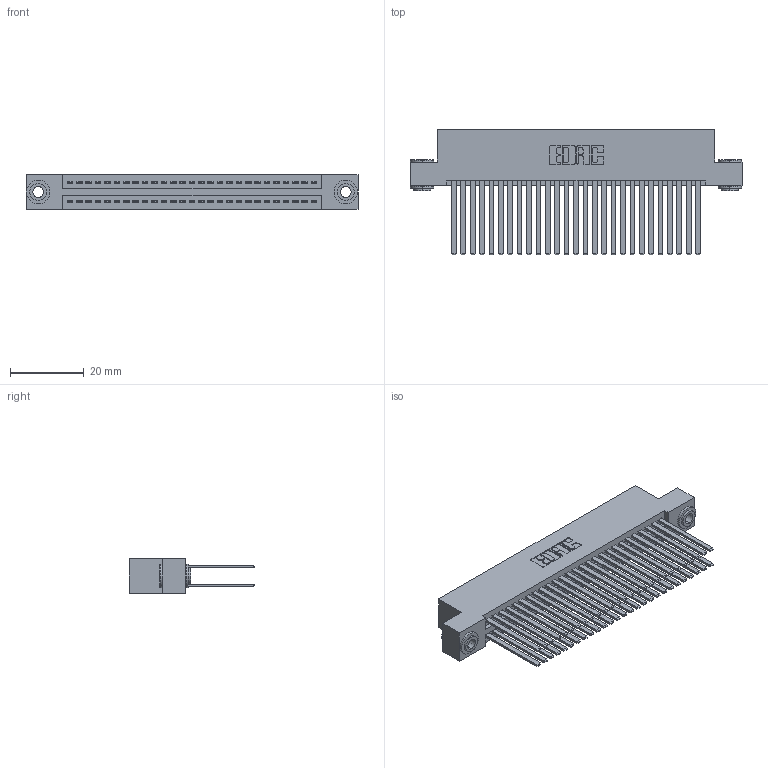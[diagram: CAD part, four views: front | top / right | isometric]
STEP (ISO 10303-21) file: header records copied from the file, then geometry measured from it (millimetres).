
FILE_DESCRIPTION (( 'STEP AP203' ), '1' );
FILE_NAME ('395-054-544-203.STEP', '2019-10-19T17:10:13', ( '' ), ( '' ), 'SwSTEP 2.0', 'SolidWorks 2016', '' );
FILE_SCHEMA (( 'CONFIG_CONTROL_DESIGN' ));
Length unit declared in the file: inch
Products named in the file (4): 345 Part_Flush Mounting Lugs - 0.156 Dia-TH; 345-292-001_345-293-144; 345-250-002_345-250-002-102; 395-054-544-203
Assembly tree (57 placements, depth 2):
  395-054-544-203
    345 Part_Flush Mounting Lugs - 0.156 Dia-TH
    345-292-001_345-293-144  x54
    345-250-002_345-250-002-102  x2
Bounding box: 89.79 x 33.96 x 9.4 mm (x, y, z)
Volume: 9359.3 mm3; surface area: 15967.7 mm2
Topology: 57 solids, 57 shells, 2540 faces, 7491 edges, 4918 vertices
Faces by surface type: plane 1656, cylinder 876, cone 8
Entity records: 23670 total; most frequent: CARTESIAN_POINT 3955, ORIENTED_EDGE 3882, DIRECTION 3535, EDGE_CURVE 1941, VECTOR 1681, LINE 1681, VERTEX_POINT 1290, AXIS2_PLACEMENT_3D 927
